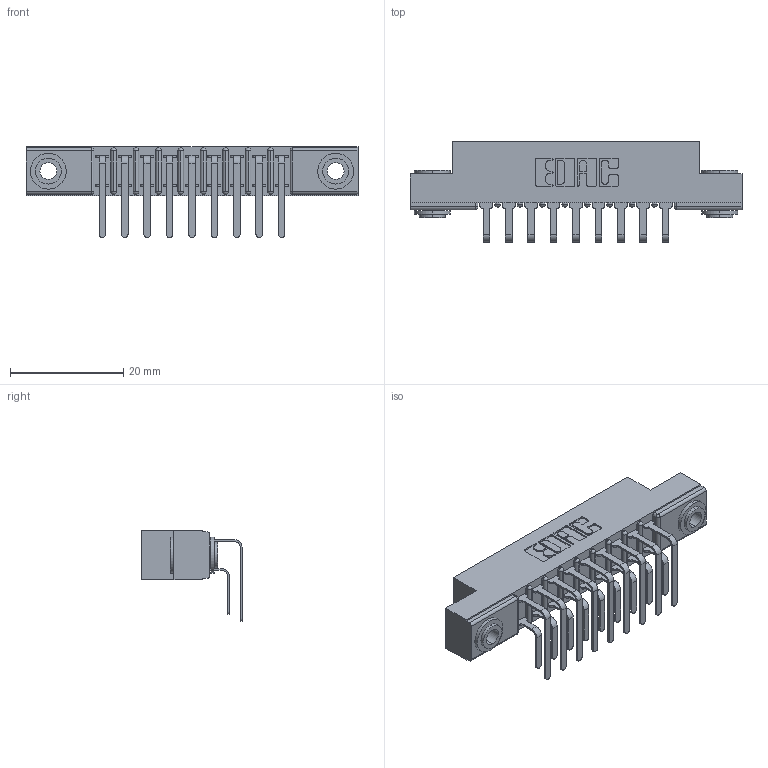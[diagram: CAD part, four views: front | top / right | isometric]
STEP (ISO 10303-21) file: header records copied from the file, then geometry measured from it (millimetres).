
FILE_DESCRIPTION (( 'STEP AP203' ), '1' );
FILE_NAME ('357-009-459-103.STEP', '2020-09-30T05:36:29', ( '' ), ( '' ), 'SwSTEP 2.0', 'SolidWorks 2020', '' );
FILE_SCHEMA (( 'CONFIG_CONTROL_DESIGN' ));
Length unit declared in the file: inch
Products named in the file (5): 345-250-002_345-250-002-102; 357-009-459-103; 307-290-001_559 - 2 (Single); 307 Part_.156 Dia Mounting Holes; 307-290-001_558 559 - 1 (Single)
Assembly tree (21 placements, depth 2):
  357-009-459-103
    307 Part_.156 Dia Mounting Holes
    307-290-001_558 559 - 1 (Single)  x9
    307-290-001_559 - 2 (Single)  x9
    345-250-002_345-250-002-102  x2
Bounding box: 58.67 x 17.69 x 16.08 mm (x, y, z)
Volume: 3920.5 mm3; surface area: 6943.1 mm2
Topology: 21 solids, 21 shells, 1080 faces, 2991 edges, 1938 vertices
Faces by surface type: plane 688, cylinder 364, sphere 20, cone 8
Entity records: 14584 total; most frequent: CARTESIAN_POINT 2380, DIRECTION 2359, ORIENTED_EDGE 2346, EDGE_CURVE 1173, VECTOR 877, LINE 877, VERTEX_POINT 762, AXIS2_PLACEMENT_3D 741
